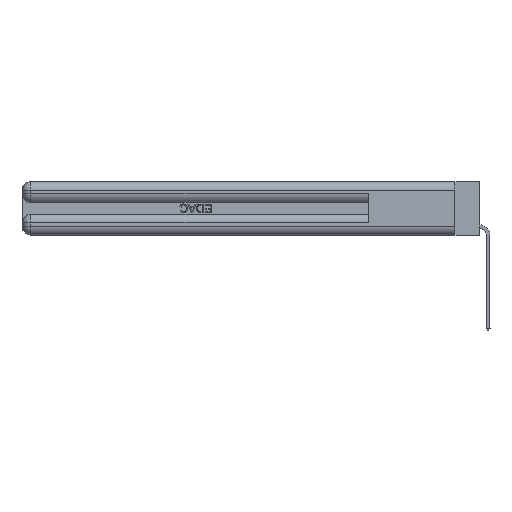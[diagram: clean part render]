
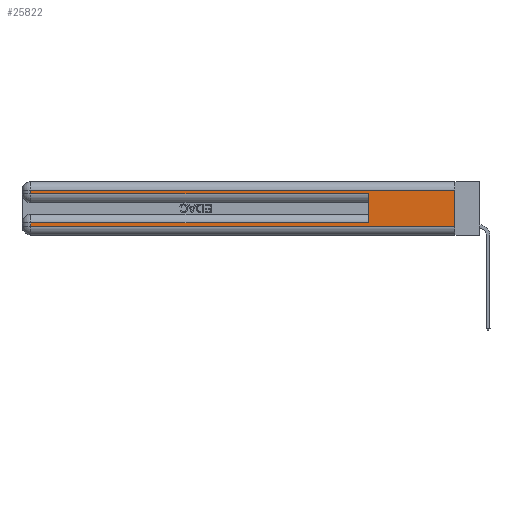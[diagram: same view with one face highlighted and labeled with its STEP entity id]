
A CAD part, left-side view. The second image highlights one B-rep face of the part: STEP entity #25822.
In plain terms, the highlighted planar face has unit normal (-1, 0, 0).
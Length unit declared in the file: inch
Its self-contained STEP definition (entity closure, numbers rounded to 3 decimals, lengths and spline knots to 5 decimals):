
#173 = CARTESIAN_POINT ( 'NONE',  ( 0., 2.94, 0.285 ) ) ;
#572 = ORIENTED_EDGE ( 'NONE', *, *, #17960, .T. ) ;
#600 = CARTESIAN_POINT ( 'NONE',  ( 0., 2.94, 0.37 ) ) ;
#862 = DIRECTION ( 'NONE',  ( 0., 0., -1. ) ) ;
#1016 = EDGE_CURVE ( 'NONE', #32453, #2167, #10184, .T. ) ;
#1682 = EDGE_CURVE ( 'NONE', #3041, #30928, #13382, .T. ) ;
#2053 = EDGE_LOOP ( 'NONE', ( #6926, #572, #10882, #4638, #16036, #7863, #18409, #6910 ) ) ;
#2140 = CARTESIAN_POINT ( 'NONE',  ( 0., 0.6, 0.085 ) ) ;
#2167 = VERTEX_POINT ( 'NONE', #11108 ) ;
#3041 = VERTEX_POINT ( 'NONE', #173 ) ;
#3342 = DIRECTION ( 'NONE',  ( 0., 0., -1. ) ) ;
#4638 = ORIENTED_EDGE ( 'NONE', *, *, #1682, .T. ) ;
#5780 = VERTEX_POINT ( 'NONE', #2140 ) ;
#5831 = CARTESIAN_POINT ( 'NONE',  ( 0., 0.6, 0.285 ) ) ;
#6107 = DIRECTION ( 'NONE',  ( 0., 1., 0. ) ) ;
#6332 = PLANE ( 'NONE',  #12465 ) ;
#6910 = ORIENTED_EDGE ( 'NONE', *, *, #1016, .T. ) ;
#6926 = ORIENTED_EDGE ( 'NONE', *, *, #27998, .F. ) ;
#7616 = CARTESIAN_POINT ( 'NONE',  ( 0., 2.94, 0.37 ) ) ;
#7863 = ORIENTED_EDGE ( 'NONE', *, *, #18067, .T. ) ;
#9296 = VECTOR ( 'NONE', #16364, 39.37008 ) ;
#9338 = LINE ( 'NONE', #19135, #9729 ) ;
#9728 = VECTOR ( 'NONE', #26113, 39.37008 ) ;
#9729 = VECTOR ( 'NONE', #30053, 39.37008 ) ;
#10181 = VERTEX_POINT ( 'NONE', #10237 ) ;
#10184 = LINE ( 'NONE', #25937, #9728 ) ;
#10237 = CARTESIAN_POINT ( 'NONE',  ( 0., 0., 0.31 ) ) ;
#10882 = ORIENTED_EDGE ( 'NONE', *, *, #23561, .T. ) ;
#11108 = CARTESIAN_POINT ( 'NONE',  ( 0., 0., 0.06 ) ) ;
#11586 = VECTOR ( 'NONE', #6107, 39.37008 ) ;
#12465 = AXIS2_PLACEMENT_3D ( 'NONE', #19533, #32362, #862 ) ;
#13382 = LINE ( 'NONE', #16627, #17440 ) ;
#15293 = VERTEX_POINT ( 'NONE', #28191 ) ;
#16036 = ORIENTED_EDGE ( 'NONE', *, *, #26491, .F. ) ;
#16364 = DIRECTION ( 'NONE',  ( 0., 0., -1. ) ) ;
#16627 = CARTESIAN_POINT ( 'NONE',  ( 0., 0., 0.285 ) ) ;
#17440 = VECTOR ( 'NONE', #26738, 39.37008 ) ;
#17960 = EDGE_CURVE ( 'NONE', #10181, #15293, #18982, .T. ) ;
#18067 = EDGE_CURVE ( 'NONE', #5780, #26660, #32472, .T. ) ;
#18409 = ORIENTED_EDGE ( 'NONE', *, *, #18749, .T. ) ;
#18749 = EDGE_CURVE ( 'NONE', #26660, #32453, #31590, .T. ) ;
#18982 = LINE ( 'NONE', #29569, #11586 ) ;
#19135 = CARTESIAN_POINT ( 'NONE',  ( 0., 0.6, 0.145 ) ) ;
#19197 = FACE_OUTER_BOUND ( 'NONE', #2053, .T. ) ;
#19533 = CARTESIAN_POINT ( 'NONE',  ( 0., 0., 0.37 ) ) ;
#19817 = CARTESIAN_POINT ( 'NONE',  ( 0., 0., 0.085 ) ) ;
#20376 = VECTOR ( 'NONE', #27171, 39.37008 ) ;
#20967 = VECTOR ( 'NONE', #28855, 39.37008 ) ;
#21648 = CARTESIAN_POINT ( 'NONE',  ( 0., 2.94, 0.06 ) ) ;
#21682 = CARTESIAN_POINT ( 'NONE',  ( 0., 0., 0.37 ) ) ;
#22899 = CARTESIAN_POINT ( 'NONE',  ( 0., 2.94, 0.085 ) ) ;
#23561 = EDGE_CURVE ( 'NONE', #15293, #3041, #23919, .T. ) ;
#23919 = LINE ( 'NONE', #600, #28207 ) ;
#25822 = ADVANCED_FACE ( 'NONE', ( #19197 ), #6332, .F. ) ;
#25937 = CARTESIAN_POINT ( 'NONE',  ( 0., 0., 0.06 ) ) ;
#26113 = DIRECTION ( 'NONE',  ( 0., -1., 0. ) ) ;
#26491 = EDGE_CURVE ( 'NONE', #5780, #30928, #9338, .T. ) ;
#26660 = VERTEX_POINT ( 'NONE', #22899 ) ;
#26738 = DIRECTION ( 'NONE',  ( 0., -1., 0. ) ) ;
#27171 = DIRECTION ( 'NONE',  ( 0., 1., 0. ) ) ;
#27998 = EDGE_CURVE ( 'NONE', #10181, #2167, #31440, .T. ) ;
#28191 = CARTESIAN_POINT ( 'NONE',  ( 0., 2.94, 0.31 ) ) ;
#28207 = VECTOR ( 'NONE', #3342, 39.37008 ) ;
#28855 = DIRECTION ( 'NONE',  ( 0., 0., -1. ) ) ;
#29569 = CARTESIAN_POINT ( 'NONE',  ( 0., 0., 0.31 ) ) ;
#30053 = DIRECTION ( 'NONE',  ( 0., 0., 1. ) ) ;
#30928 = VERTEX_POINT ( 'NONE', #5831 ) ;
#31440 = LINE ( 'NONE', #21682, #9296 ) ;
#31590 = LINE ( 'NONE', #7616, #20967 ) ;
#32362 = DIRECTION ( 'NONE',  ( 1., 0., 0. ) ) ;
#32453 = VERTEX_POINT ( 'NONE', #21648 ) ;
#32472 = LINE ( 'NONE', #19817, #20376 ) ;
